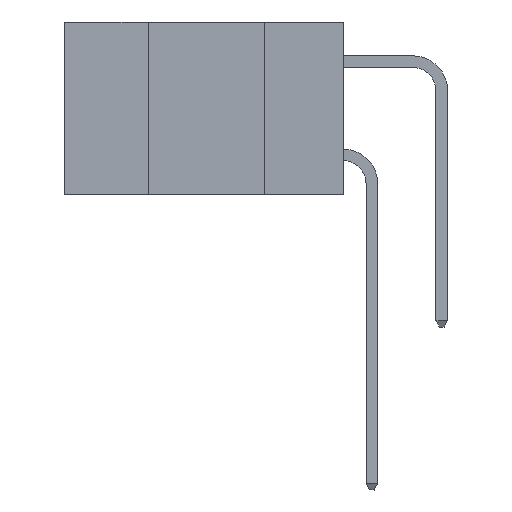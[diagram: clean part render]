
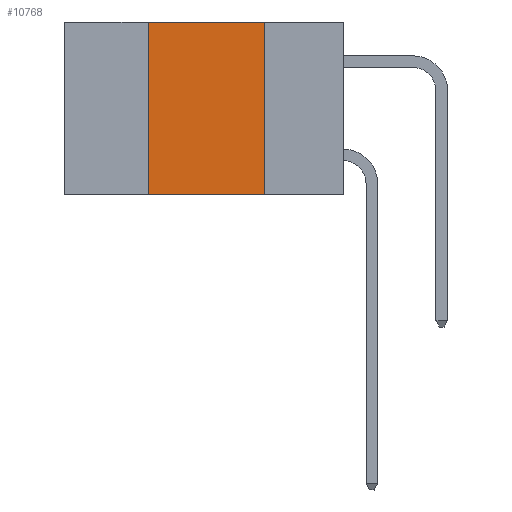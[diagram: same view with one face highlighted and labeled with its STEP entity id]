
A CAD part, left-side view. The second image highlights one B-rep face of the part: STEP entity #10768.
In plain terms, the highlighted planar face has unit normal (-1, 0, 0).
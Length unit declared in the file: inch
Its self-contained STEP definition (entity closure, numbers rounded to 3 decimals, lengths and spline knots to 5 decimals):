
#427 = CARTESIAN_POINT ( 'NONE',  ( 0., 0.6, 0. ) ) ;
#708 = CARTESIAN_POINT ( 'NONE',  ( 0., 0.42, -0.37 ) ) ;
#1011 = LINE ( 'NONE', #5964, #4025 ) ;
#1217 = DIRECTION ( 'NONE',  ( 0., 0., -1. ) ) ;
#2183 = CARTESIAN_POINT ( 'NONE',  ( 0., 0.17, -0.37 ) ) ;
#2597 = VERTEX_POINT ( 'NONE', #9190 ) ;
#2621 = FACE_OUTER_BOUND ( 'NONE', #4713, .T. ) ;
#3595 = EDGE_CURVE ( 'NONE', #3749, #2597, #12128, .T. ) ;
#3749 = VERTEX_POINT ( 'NONE', #5509 ) ;
#4003 = VECTOR ( 'NONE', #10292, 39.37008 ) ;
#4025 = VECTOR ( 'NONE', #12629, 39.37008 ) ;
#4209 = VECTOR ( 'NONE', #1217, 39.37008 ) ;
#4373 = DIRECTION ( 'NONE',  ( 0., -1., 0. ) ) ;
#4474 = VERTEX_POINT ( 'NONE', #6257 ) ;
#4713 = EDGE_LOOP ( 'NONE', ( #5678, #6241, #12099, #11678 ) ) ;
#5151 = LINE ( 'NONE', #2183, #4209 ) ;
#5509 = CARTESIAN_POINT ( 'NONE',  ( 0., 0.42, 0. ) ) ;
#5678 = ORIENTED_EDGE ( 'NONE', *, *, #6544, .F. ) ;
#5964 = CARTESIAN_POINT ( 'NONE',  ( 0., 0.6, -0.37 ) ) ;
#6241 = ORIENTED_EDGE ( 'NONE', *, *, #3595, .F. ) ;
#6257 = CARTESIAN_POINT ( 'NONE',  ( 0., 0.42, -0.37 ) ) ;
#6383 = LINE ( 'NONE', #708, #4003 ) ;
#6520 = CARTESIAN_POINT ( 'NONE',  ( 0., 0.17, -0.37 ) ) ;
#6544 = EDGE_CURVE ( 'NONE', #2597, #9376, #5151, .T. ) ;
#6592 = CARTESIAN_POINT ( 'NONE',  ( 0., 0.6, 0. ) ) ;
#7139 = EDGE_CURVE ( 'NONE', #4474, #3749, #6383, .T. ) ;
#7511 = DIRECTION ( 'NONE',  ( 1., 0., 0. ) ) ;
#7772 = PLANE ( 'NONE',  #10129 ) ;
#9190 = CARTESIAN_POINT ( 'NONE',  ( 0., 0.17, 0. ) ) ;
#9376 = VERTEX_POINT ( 'NONE', #6520 ) ;
#9763 = VECTOR ( 'NONE', #4373, 39.37008 ) ;
#10129 = AXIS2_PLACEMENT_3D ( 'NONE', #6592, #7511, #11395 ) ;
#10292 = DIRECTION ( 'NONE',  ( 0., 0., 1. ) ) ;
#10768 = ADVANCED_FACE ( 'NONE', ( #2621 ), #7772, .F. ) ;
#11395 = DIRECTION ( 'NONE',  ( 0., 0., -1. ) ) ;
#11678 = ORIENTED_EDGE ( 'NONE', *, *, #12205, .T. ) ;
#12099 = ORIENTED_EDGE ( 'NONE', *, *, #7139, .F. ) ;
#12128 = LINE ( 'NONE', #427, #9763 ) ;
#12205 = EDGE_CURVE ( 'NONE', #4474, #9376, #1011, .T. ) ;
#12629 = DIRECTION ( 'NONE',  ( 0., -1., 0. ) ) ;
